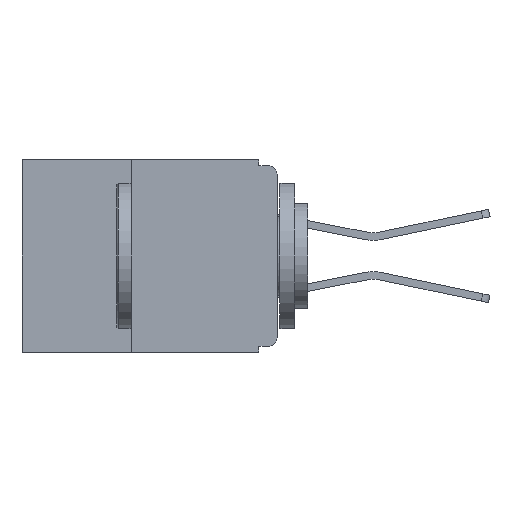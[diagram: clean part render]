
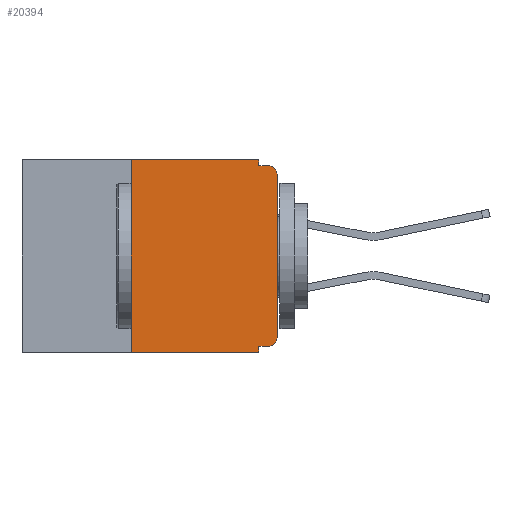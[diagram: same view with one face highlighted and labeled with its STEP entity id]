
A CAD part, left-side view. The second image highlights one B-rep face of the part: STEP entity #20394.
In plain terms, the highlighted planar face has unit normal (-1, 0, 0).
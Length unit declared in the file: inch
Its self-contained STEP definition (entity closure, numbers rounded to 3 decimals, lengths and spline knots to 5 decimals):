
#37 = VERTEX_POINT ( 'NONE', #741 ) ;
#191 = VECTOR ( 'NONE', #3371, 39.37008 ) ;
#263 = LINE ( 'NONE', #13826, #8512 ) ;
#726 = CARTESIAN_POINT ( 'NONE',  ( 0., 0.25, 0. ) ) ;
#741 = CARTESIAN_POINT ( 'NONE',  ( 0., 0., -0.025 ) ) ;
#785 = VERTEX_POINT ( 'NONE', #21012 ) ;
#1224 = EDGE_CURVE ( 'NONE', #11828, #11760, #263, .T. ) ;
#1831 = EDGE_CURVE ( 'NONE', #5143, #785, #19949, .T. ) ;
#2132 = CARTESIAN_POINT ( 'NONE',  ( 0., 0.015, -0.025 ) ) ;
#2464 = AXIS2_PLACEMENT_3D ( 'NONE', #15939, #5286, #17707 ) ;
#3018 = PLANE ( 'NONE',  #5915 ) ;
#3216 = ORIENTED_EDGE ( 'NONE', *, *, #12905, .T. ) ;
#3371 = DIRECTION ( 'NONE',  ( 0., -1., 0. ) ) ;
#3560 = CARTESIAN_POINT ( 'NONE',  ( 0., 0.031, -0.33 ) ) ;
#3871 = DIRECTION ( 'NONE',  ( 0., 0., -1. ) ) ;
#4106 = CARTESIAN_POINT ( 'NONE',  ( 0., 0.031, 0. ) ) ;
#4139 = CARTESIAN_POINT ( 'NONE',  ( 0., 0.031, -0.32 ) ) ;
#4483 = FACE_OUTER_BOUND ( 'NONE', #17075, .T. ) ;
#4732 = EDGE_CURVE ( 'NONE', #13507, #11828, #20950, .T. ) ;
#4776 = CARTESIAN_POINT ( 'NONE',  ( 0., 0.437, 0. ) ) ;
#4904 = LINE ( 'NONE', #10370, #191 ) ;
#5143 = VERTEX_POINT ( 'NONE', #6945 ) ;
#5286 = DIRECTION ( 'NONE',  ( -1., 0., 0. ) ) ;
#5661 = ORIENTED_EDGE ( 'NONE', *, *, #1831, .F. ) ;
#5897 = EDGE_CURVE ( 'NONE', #11760, #5143, #14532, .T. ) ;
#5915 = AXIS2_PLACEMENT_3D ( 'NONE', #4776, #17170, #6521 ) ;
#5994 = CARTESIAN_POINT ( 'NONE',  ( 0., 0.031, -0.33 ) ) ;
#6521 = DIRECTION ( 'NONE',  ( 0., 0., -1. ) ) ;
#6755 = ORIENTED_EDGE ( 'NONE', *, *, #4732, .F. ) ;
#6945 = CARTESIAN_POINT ( 'NONE',  ( 0., 0.031, -0.01 ) ) ;
#7475 = DIRECTION ( 'NONE',  ( 0., 0., 1. ) ) ;
#7527 = CARTESIAN_POINT ( 'NONE',  ( 0., 0., -0.305 ) ) ;
#7700 = CIRCLE ( 'NONE', #21534, 0.015 ) ;
#8391 = VECTOR ( 'NONE', #8590, 39.37008 ) ;
#8512 = VECTOR ( 'NONE', #13855, 39.37008 ) ;
#8590 = DIRECTION ( 'NONE',  ( 0., 1., 0. ) ) ;
#8841 = EDGE_CURVE ( 'NONE', #12438, #37, #21398, .T. ) ;
#9073 = CARTESIAN_POINT ( 'NONE',  ( 0., 0.25, -0.33 ) ) ;
#9240 = CARTESIAN_POINT ( 'NONE',  ( 0., 0., -0.01 ) ) ;
#10370 = CARTESIAN_POINT ( 'NONE',  ( 0., 0.437, -0.33 ) ) ;
#10456 = VECTOR ( 'NONE', #12217, 39.37008 ) ;
#11274 = EDGE_CURVE ( 'NONE', #13507, #22041, #4904, .T. ) ;
#11298 = CARTESIAN_POINT ( 'NONE',  ( 0., 0.015, -0.32 ) ) ;
#11371 = DIRECTION ( 'NONE',  ( 0., 0., 1. ) ) ;
#11443 = VECTOR ( 'NONE', #11371, 39.37008 ) ;
#11503 = ORIENTED_EDGE ( 'NONE', *, *, #11274, .T. ) ;
#11569 = CARTESIAN_POINT ( 'NONE',  ( 0., 0.25, -0.33 ) ) ;
#11760 = VERTEX_POINT ( 'NONE', #4106 ) ;
#11827 = VERTEX_POINT ( 'NONE', #11298 ) ;
#11828 = VERTEX_POINT ( 'NONE', #726 ) ;
#12073 = ORIENTED_EDGE ( 'NONE', *, *, #21860, .F. ) ;
#12217 = DIRECTION ( 'NONE',  ( 0., -1., 0. ) ) ;
#12438 = VERTEX_POINT ( 'NONE', #7527 ) ;
#12604 = LINE ( 'NONE', #19291, #8391 ) ;
#12905 = EDGE_CURVE ( 'NONE', #11827, #12438, #21258, .T. ) ;
#13320 = CARTESIAN_POINT ( 'NONE',  ( 0., 0.031, 0. ) ) ;
#13452 = ORIENTED_EDGE ( 'NONE', *, *, #8841, .T. ) ;
#13507 = VERTEX_POINT ( 'NONE', #9073 ) ;
#13826 = CARTESIAN_POINT ( 'NONE',  ( 0., 0.437, 0. ) ) ;
#13855 = DIRECTION ( 'NONE',  ( 0., -1., 0. ) ) ;
#13986 = VECTOR ( 'NONE', #16216, 39.37008 ) ;
#14481 = DIRECTION ( 'NONE',  ( -1., 0., 0. ) ) ;
#14532 = LINE ( 'NONE', #13320, #13986 ) ;
#14555 = CARTESIAN_POINT ( 'NONE',  ( 0., 0., 0. ) ) ;
#15124 = ORIENTED_EDGE ( 'NONE', *, *, #5897, .F. ) ;
#15313 = EDGE_CURVE ( 'NONE', #37, #785, #7700, .T. ) ;
#15939 = CARTESIAN_POINT ( 'NONE',  ( 0., 0.015, -0.305 ) ) ;
#16216 = DIRECTION ( 'NONE',  ( 0., 0., -1. ) ) ;
#16339 = LINE ( 'NONE', #3560, #20545 ) ;
#16627 = VECTOR ( 'NONE', #7475, 39.37008 ) ;
#17075 = EDGE_LOOP ( 'NONE', ( #13452, #18724, #5661, #15124, #19853, #6755, #11503, #12073, #21553, #3216 ) ) ;
#17170 = DIRECTION ( 'NONE',  ( 1., 0., 0. ) ) ;
#17678 = EDGE_CURVE ( 'NONE', #11827, #22638, #12604, .T. ) ;
#17707 = DIRECTION ( 'NONE',  ( 0., 0., -1. ) ) ;
#17817 = DIRECTION ( 'NONE',  ( 0., 0., -1. ) ) ;
#18724 = ORIENTED_EDGE ( 'NONE', *, *, #15313, .T. ) ;
#19291 = CARTESIAN_POINT ( 'NONE',  ( 0., 0., -0.32 ) ) ;
#19853 = ORIENTED_EDGE ( 'NONE', *, *, #1224, .F. ) ;
#19949 = LINE ( 'NONE', #9240, #10456 ) ;
#20394 = ADVANCED_FACE ( 'NONE', ( #4483 ), #3018, .F. ) ;
#20545 = VECTOR ( 'NONE', #17817, 39.37008 ) ;
#20950 = LINE ( 'NONE', #11569, #11443 ) ;
#21012 = CARTESIAN_POINT ( 'NONE',  ( 0., 0.015, -0.01 ) ) ;
#21258 = CIRCLE ( 'NONE', #2464, 0.015 ) ;
#21398 = LINE ( 'NONE', #14555, #16627 ) ;
#21534 = AXIS2_PLACEMENT_3D ( 'NONE', #2132, #14481, #3871 ) ;
#21553 = ORIENTED_EDGE ( 'NONE', *, *, #17678, .F. ) ;
#21860 = EDGE_CURVE ( 'NONE', #22638, #22041, #16339, .T. ) ;
#22041 = VERTEX_POINT ( 'NONE', #5994 ) ;
#22638 = VERTEX_POINT ( 'NONE', #4139 ) ;
